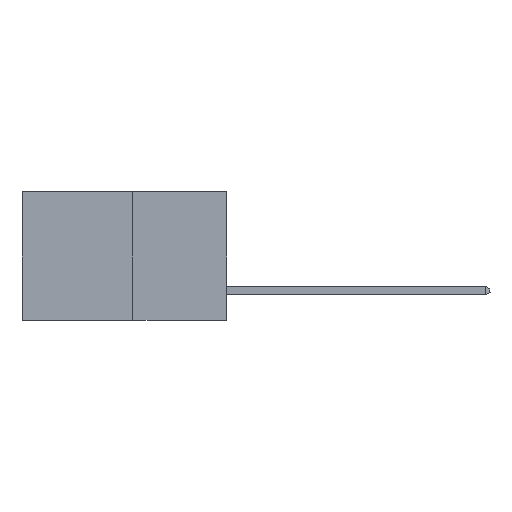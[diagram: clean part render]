
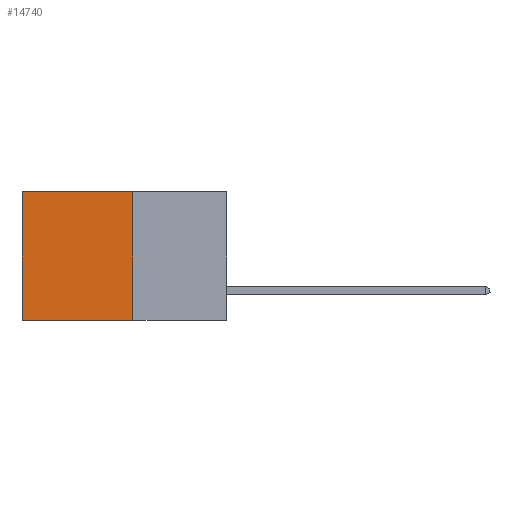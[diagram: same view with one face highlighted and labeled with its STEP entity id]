
A CAD part, left-side view. The second image highlights one B-rep face of the part: STEP entity #14740.
In plain terms, the highlighted planar face has unit normal (-1, 0, 0).
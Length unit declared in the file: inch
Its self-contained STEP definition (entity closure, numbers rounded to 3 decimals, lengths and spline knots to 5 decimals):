
#112 = VERTEX_POINT ( 'NONE', #15566 ) ;
#866 = LINE ( 'NONE', #9657, #12190 ) ;
#1921 = CARTESIAN_POINT ( 'NONE',  ( 0.277, 0.59, 0. ) ) ;
#2846 = FACE_OUTER_BOUND ( 'NONE', #9157, .T. ) ;
#2858 = EDGE_CURVE ( 'NONE', #7162, #4855, #10961, .T. ) ;
#3446 = ORIENTED_EDGE ( 'NONE', *, *, #10608, .T. ) ;
#4505 = DIRECTION ( 'NONE',  ( 0., 0., -1. ) ) ;
#4855 = VERTEX_POINT ( 'NONE', #1921 ) ;
#6205 = DIRECTION ( 'NONE',  ( 1., 0., 0. ) ) ;
#6394 = CARTESIAN_POINT ( 'NONE',  ( 0.277, 0.27, -0.37 ) ) ;
#6501 = VECTOR ( 'NONE', #4505, 39.37008 ) ;
#7162 = VERTEX_POINT ( 'NONE', #9320 ) ;
#7614 = ORIENTED_EDGE ( 'NONE', *, *, #11313, .F. ) ;
#7840 = ORIENTED_EDGE ( 'NONE', *, *, #18086, .F. ) ;
#9157 = EDGE_LOOP ( 'NONE', ( #3446, #7840, #7614, #11541 ) ) ;
#9320 = CARTESIAN_POINT ( 'NONE',  ( 0.277, 0.27, 0. ) ) ;
#9657 = CARTESIAN_POINT ( 'NONE',  ( 0.277, 0.27, -0.37 ) ) ;
#10608 = EDGE_CURVE ( 'NONE', #4855, #112, #12275, .T. ) ;
#10961 = LINE ( 'NONE', #14315, #14344 ) ;
#11131 = DIRECTION ( 'NONE',  ( 0., 1., 0. ) ) ;
#11313 = EDGE_CURVE ( 'NONE', #7162, #13993, #14479, .T. ) ;
#11541 = ORIENTED_EDGE ( 'NONE', *, *, #2858, .T. ) ;
#11568 = CARTESIAN_POINT ( 'NONE',  ( 0.277, 0.27, -0.37 ) ) ;
#12045 = PLANE ( 'NONE',  #14876 ) ;
#12190 = VECTOR ( 'NONE', #11131, 39.37008 ) ;
#12275 = LINE ( 'NONE', #17541, #6501 ) ;
#12898 = DIRECTION ( 'NONE',  ( 0., 1., 0. ) ) ;
#13483 = CARTESIAN_POINT ( 'NONE',  ( 0.277, 0.27, -0.37 ) ) ;
#13678 = DIRECTION ( 'NONE',  ( 0., 0., -1. ) ) ;
#13993 = VERTEX_POINT ( 'NONE', #11568 ) ;
#14315 = CARTESIAN_POINT ( 'NONE',  ( 0.277, 0.27, 0. ) ) ;
#14344 = VECTOR ( 'NONE', #12898, 39.37008 ) ;
#14479 = LINE ( 'NONE', #6394, #18332 ) ;
#14740 = ADVANCED_FACE ( 'NONE', ( #2846 ), #12045, .F. ) ;
#14876 = AXIS2_PLACEMENT_3D ( 'NONE', #13483, #6205, #16387 ) ;
#15566 = CARTESIAN_POINT ( 'NONE',  ( 0.277, 0.59, -0.37 ) ) ;
#16387 = DIRECTION ( 'NONE',  ( 0., 0., -1. ) ) ;
#17541 = CARTESIAN_POINT ( 'NONE',  ( 0.277, 0.59, -0.37 ) ) ;
#18086 = EDGE_CURVE ( 'NONE', #13993, #112, #866, .T. ) ;
#18332 = VECTOR ( 'NONE', #13678, 39.37008 ) ;
